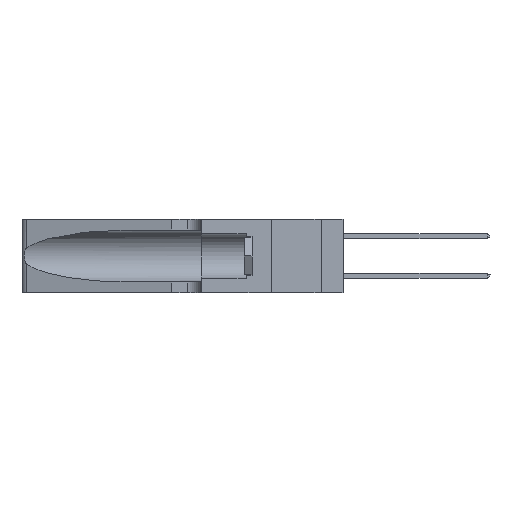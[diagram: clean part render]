
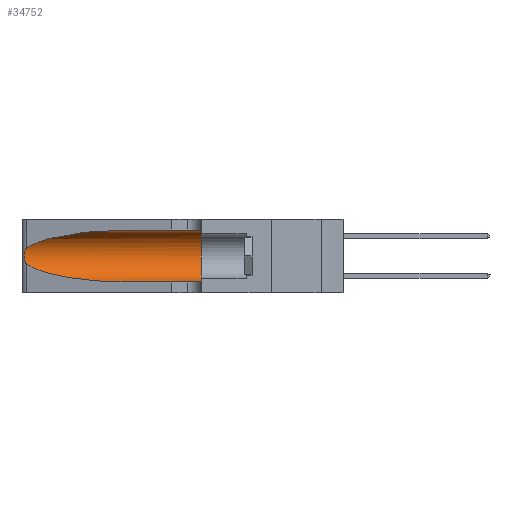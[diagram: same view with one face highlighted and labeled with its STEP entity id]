
A CAD part, left-side view. The second image highlights one B-rep face of the part: STEP entity #34752.
In plain terms, the highlighted cylindrical face has radius 3.308 mm (diameter 6.617 mm), a partial arc.
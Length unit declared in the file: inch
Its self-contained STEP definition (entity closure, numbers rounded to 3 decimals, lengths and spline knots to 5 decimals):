
#810 = CARTESIAN_POINT ( 'NONE',  ( 0.25487, 1.22718, 0.22369 ) ) ;
#1752 = CARTESIAN_POINT ( 'NONE',  ( 0.25639, 1.23186, 0.15144 ) ) ;
#2223 = EDGE_LOOP ( 'NONE', ( #13461, #16236, #25673, #21267, #5832, #34113 ) ) ;
#2300 = LINE ( 'NONE', #23450, #29486 ) ;
#2641 = CARTESIAN_POINT ( 'NONE',  ( 0.1305, 0.35, 0.05475 ) ) ;
#5179 = CARTESIAN_POINT ( 'NONE',  ( 0.25487, 1.22718, 0.22369 ) ) ;
#5331 = CARTESIAN_POINT ( 'NONE',  ( 0.25487, 1.22718, 0.14631 ) ) ;
#5832 = ORIENTED_EDGE ( 'NONE', *, *, #30764, .F. ) ;
#8754 = CARTESIAN_POINT ( 'NONE',  ( 0.25639, 1.23184, 0.21858 ) ) ;
#9079 = CARTESIAN_POINT ( 'NONE',  ( 0.1305, 0.72297, 0.05475 ) ) ;
#10443 = VERTEX_POINT ( 'NONE', #9079 ) ;
#11202 = EDGE_CURVE ( 'NONE', #21779, #22486, #20978, .T. ) ;
#11344 = CIRCLE ( 'NONE', #12490, 0.13025 ) ;
#11721 = CARTESIAN_POINT ( 'NONE',  ( 0.1305, 0.35, 0.31525 ) ) ;
#11986 = DIRECTION ( 'NONE',  ( 0., -1., 0. ) ) ;
#12314 = CARTESIAN_POINT ( 'NONE',  ( 0.25854, 1.2359, 0.20912 ) ) ;
#12490 = AXIS2_PLACEMENT_3D ( 'NONE', #18960, #43551, #22521 ) ;
#12931 = DIRECTION ( 'NONE',  ( 0., -1., 0. ) ) ;
#13364 = EDGE_CURVE ( 'NONE', #21779, #22562, #2300, .T. ) ;
#13461 = ORIENTED_EDGE ( 'NONE', *, *, #11202, .T. ) ;
#15402 = CARTESIAN_POINT ( 'NONE',  ( 0.18966, 0.96281, 0.05475 ) ) ;
#15872 = CARTESIAN_POINT ( 'NONE',  ( 0.26075, 1.23896, 0.19203 ) ) ;
#16236 = ORIENTED_EDGE ( 'NONE', *, *, #30839, .T. ) ;
#18797 = CARTESIAN_POINT ( 'NONE',  ( 0.2373, 1.15595, 0.08982 ) ) ;
#18960 = CARTESIAN_POINT ( 'NONE',  ( 0.1305, 0.35, 0.185 ) ) ;
#19085 = CARTESIAN_POINT ( 'NONE',  ( 0.1305, 1.61858, 0.185 ) ) ;
#19421 = CARTESIAN_POINT ( 'NONE',  ( 0.26017, 1.23833, 0.17102 ) ) ;
#20281 = CARTESIAN_POINT ( 'NONE',  ( 0.1305, 0.72297, 0.31525 ) ) ;
#20978 =( BOUNDED_CURVE ( )  B_SPLINE_CURVE ( 3, ( #20281, #41371, #44842, #23865 ),
 .UNSPECIFIED., .F., .F. ) 
 B_SPLINE_CURVE_WITH_KNOTS ( ( 4, 4 ),
 ( 1.5708, 2.84003 ),
 .UNSPECIFIED. ) 
 CURVE ( )  GEOMETRIC_REPRESENTATION_ITEM ( )  RATIONAL_B_SPLINE_CURVE ( ( 1., 0.87, 0.87, 1. ) ) 
 REPRESENTATION_ITEM ( '' )  );
#21267 = ORIENTED_EDGE ( 'NONE', *, *, #44867, .T. ) ;
#21779 = VERTEX_POINT ( 'NONE', #43007 ) ;
#21886 = CARTESIAN_POINT ( 'NONE',  ( 0.1305, 1.61858, 0.05475 ) ) ;
#22359 = CARTESIAN_POINT ( 'NONE',  ( 0.25487, 1.22718, 0.14631 ) ) ;
#22486 = VERTEX_POINT ( 'NONE', #810 ) ;
#22521 = DIRECTION ( 'NONE',  ( 0., 0., 1. ) ) ;
#22562 = VERTEX_POINT ( 'NONE', #11721 ) ;
#22982 = CARTESIAN_POINT ( 'NONE',  ( 0.25789, 1.23486, 0.15765 ) ) ;
#23450 = CARTESIAN_POINT ( 'NONE',  ( 0.1305, 1.61858, 0.31525 ) ) ;
#23865 = CARTESIAN_POINT ( 'NONE',  ( 0.25487, 1.22718, 0.22369 ) ) ;
#25465 = DIRECTION ( 'NONE',  ( 0., -1., 0. ) ) ;
#25673 = ORIENTED_EDGE ( 'NONE', *, *, #32765, .T. ) ;
#25810 =( BOUNDED_CURVE ( )  B_SPLINE_CURVE ( 3, ( #22359, #18797, #15402, #40041 ),
 .UNSPECIFIED., .F., .F. ) 
 B_SPLINE_CURVE_WITH_KNOTS ( ( 4, 4 ),
 ( 3.44316, 4.71239 ),
 .UNSPECIFIED. ) 
 CURVE ( )  GEOMETRIC_REPRESENTATION_ITEM ( )  RATIONAL_B_SPLINE_CURVE ( ( 1., 0.87, 0.87, 1. ) ) 
 REPRESENTATION_ITEM ( '' )  );
#26559 = CARTESIAN_POINT ( 'NONE',  ( 0.25555, 1.22993, 0.14849 ) ) ;
#29486 = VECTOR ( 'NONE', #12931, 39.37008 ) ;
#30764 = EDGE_CURVE ( 'NONE', #22562, #35010, #11344, .T. ) ;
#30839 = EDGE_CURVE ( 'NONE', #22486, #34452, #33987, .T. ) ;
#32765 = EDGE_CURVE ( 'NONE', #34452, #10443, #25810, .T. ) ;
#33320 = CARTESIAN_POINT ( 'NONE',  ( 0.25555, 1.22994, 0.2215 ) ) ;
#33464 = CARTESIAN_POINT ( 'NONE',  ( 0.25787, 1.23484, 0.2124 ) ) ;
#33987 = B_SPLINE_CURVE_WITH_KNOTS ( 'NONE', 3,
 ( #5179, #33320, #8754, #33464, #12314, #36982, #15872, #40506, #19421, #43995, #22982, #1752, #26559, #5331 ),
 .UNSPECIFIED., .F., .F.,
 ( 4, 2, 2, 2, 2, 2, 4 ),
 ( 0., 0.00027, 0.00053, 0.00107, 0.0016, 0.00187, 0.00214 ),
 .UNSPECIFIED. ) ;
#34113 = ORIENTED_EDGE ( 'NONE', *, *, #13364, .F. ) ;
#34452 = VERTEX_POINT ( 'NONE', #45652 ) ;
#34752 = ADVANCED_FACE ( 'NONE', ( #37551 ), #35366, .F. ) ;
#35010 = VERTEX_POINT ( 'NONE', #2641 ) ;
#35366 = CYLINDRICAL_SURFACE ( 'NONE', #42761, 0.13025 ) ;
#36982 = CARTESIAN_POINT ( 'NONE',  ( 0.26018, 1.23835, 0.19895 ) ) ;
#37551 = FACE_OUTER_BOUND ( 'NONE', #2223, .T. ) ;
#40041 = CARTESIAN_POINT ( 'NONE',  ( 0.1305, 0.72297, 0.05475 ) ) ;
#40506 = CARTESIAN_POINT ( 'NONE',  ( 0.26075, 1.23896, 0.178 ) ) ;
#41371 = CARTESIAN_POINT ( 'NONE',  ( 0.18966, 0.96281, 0.31525 ) ) ;
#42761 = AXIS2_PLACEMENT_3D ( 'NONE', #19085, #11986, #43673 ) ;
#43007 = CARTESIAN_POINT ( 'NONE',  ( 0.1305, 0.72297, 0.31525 ) ) ;
#43551 = DIRECTION ( 'NONE',  ( 0., 1., 0. ) ) ;
#43590 = LINE ( 'NONE', #21886, #44663 ) ;
#43673 = DIRECTION ( 'NONE',  ( 0., 0., -1. ) ) ;
#43995 = CARTESIAN_POINT ( 'NONE',  ( 0.25856, 1.23593, 0.16098 ) ) ;
#44663 = VECTOR ( 'NONE', #25465, 39.37008 ) ;
#44842 = CARTESIAN_POINT ( 'NONE',  ( 0.2373, 1.15595, 0.28018 ) ) ;
#44867 = EDGE_CURVE ( 'NONE', #10443, #35010, #43590, .T. ) ;
#45652 = CARTESIAN_POINT ( 'NONE',  ( 0.25487, 1.22718, 0.14631 ) ) ;
